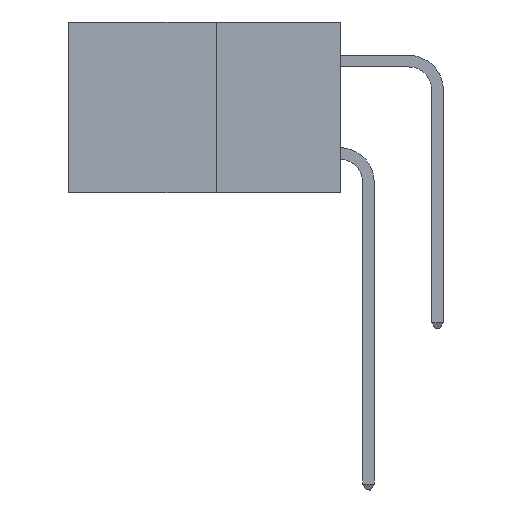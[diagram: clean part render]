
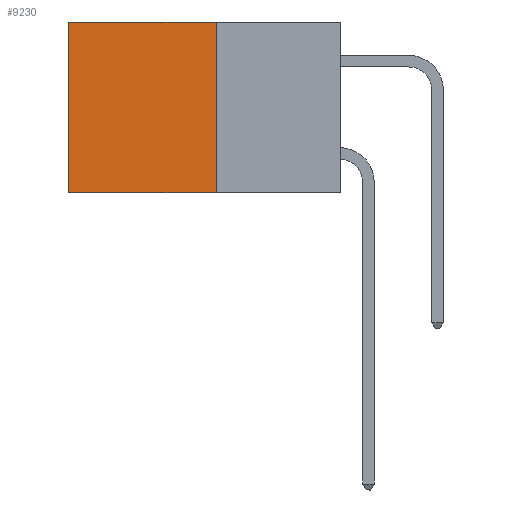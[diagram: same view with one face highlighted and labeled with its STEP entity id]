
A CAD part, left-side view. The second image highlights one B-rep face of the part: STEP entity #9230.
In plain terms, the highlighted planar face has unit normal (-1, 0, 0).
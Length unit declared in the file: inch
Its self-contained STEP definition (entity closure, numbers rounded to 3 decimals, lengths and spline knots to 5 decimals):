
#365 = EDGE_CURVE ( 'NONE', #10980, #14033, #2980, .T. ) ;
#860 = DIRECTION ( 'NONE',  ( 0., 1., 0. ) ) ;
#1575 = EDGE_LOOP ( 'NONE', ( #2252, #2823, #12926, #9626 ) ) ;
#2252 = ORIENTED_EDGE ( 'NONE', *, *, #14939, .T. ) ;
#2823 = ORIENTED_EDGE ( 'NONE', *, *, #2866, .F. ) ;
#2866 = EDGE_CURVE ( 'NONE', #14033, #8041, #5524, .T. ) ;
#2980 = LINE ( 'NONE', #17267, #10382 ) ;
#5198 = DIRECTION ( 'NONE',  ( 0., 0., -1. ) ) ;
#5524 = LINE ( 'NONE', #7909, #12471 ) ;
#6492 = CARTESIAN_POINT ( 'NONE',  ( 0.277, 0.27, -0.37 ) ) ;
#7909 = CARTESIAN_POINT ( 'NONE',  ( 0.277, 0.27, -0.37 ) ) ;
#8041 = VERTEX_POINT ( 'NONE', #13825 ) ;
#8403 = VECTOR ( 'NONE', #12590, 39.37008 ) ;
#8432 = CARTESIAN_POINT ( 'NONE',  ( 0.277, 0.59, -0.37 ) ) ;
#9230 = ADVANCED_FACE ( 'NONE', ( #15229 ), #10657, .F. ) ;
#9626 = ORIENTED_EDGE ( 'NONE', *, *, #15908, .T. ) ;
#10279 = VECTOR ( 'NONE', #15764, 39.37008 ) ;
#10382 = VECTOR ( 'NONE', #17648, 39.37008 ) ;
#10414 = AXIS2_PLACEMENT_3D ( 'NONE', #12122, #13540, #5198 ) ;
#10513 = CARTESIAN_POINT ( 'NONE',  ( 0.277, 0.27, 0. ) ) ;
#10657 = PLANE ( 'NONE',  #10414 ) ;
#10980 = VERTEX_POINT ( 'NONE', #10513 ) ;
#12073 = LINE ( 'NONE', #8432, #8403 ) ;
#12122 = CARTESIAN_POINT ( 'NONE',  ( 0.277, 0.27, -0.37 ) ) ;
#12302 = VERTEX_POINT ( 'NONE', #13231 ) ;
#12471 = VECTOR ( 'NONE', #860, 39.37008 ) ;
#12590 = DIRECTION ( 'NONE',  ( 0., 0., -1. ) ) ;
#12926 = ORIENTED_EDGE ( 'NONE', *, *, #365, .F. ) ;
#13231 = CARTESIAN_POINT ( 'NONE',  ( 0.277, 0.59, 0. ) ) ;
#13540 = DIRECTION ( 'NONE',  ( 1., 0., 0. ) ) ;
#13825 = CARTESIAN_POINT ( 'NONE',  ( 0.277, 0.59, -0.37 ) ) ;
#14009 = LINE ( 'NONE', #17102, #10279 ) ;
#14033 = VERTEX_POINT ( 'NONE', #6492 ) ;
#14939 = EDGE_CURVE ( 'NONE', #12302, #8041, #12073, .T. ) ;
#15229 = FACE_OUTER_BOUND ( 'NONE', #1575, .T. ) ;
#15764 = DIRECTION ( 'NONE',  ( 0., 1., 0. ) ) ;
#15908 = EDGE_CURVE ( 'NONE', #10980, #12302, #14009, .T. ) ;
#17102 = CARTESIAN_POINT ( 'NONE',  ( 0.277, 0.27, 0. ) ) ;
#17267 = CARTESIAN_POINT ( 'NONE',  ( 0.277, 0.27, -0.37 ) ) ;
#17648 = DIRECTION ( 'NONE',  ( 0., 0., -1. ) ) ;
